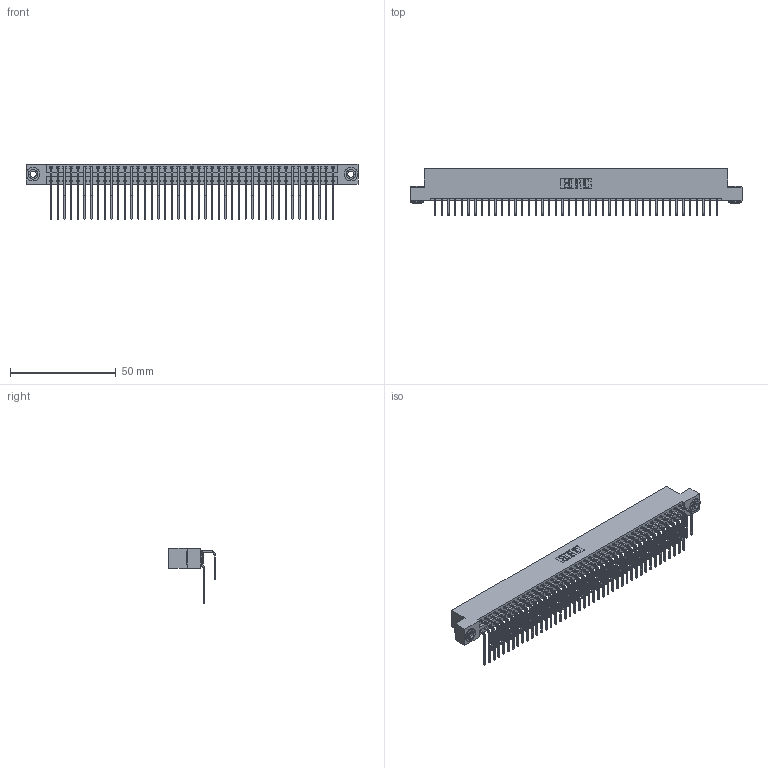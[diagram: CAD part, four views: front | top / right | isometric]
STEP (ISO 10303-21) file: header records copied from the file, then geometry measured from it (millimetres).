
FILE_DESCRIPTION (( 'STEP AP203' ), '1' );
FILE_NAME ('396-086-558-203.STEP', '2019-11-03T13:31:06', ( '' ), ( '' ), 'SwSTEP 2.0', 'SolidWorks 2016', '' );
FILE_SCHEMA (( 'CONFIG_CONTROL_DESIGN' ));
Length unit declared in the file: inch
Products named in the file (5): 345-292-001_558 Tail - 2; 345-250-002_345-250-002-102; 345-292-001_558 559 Tail - 1; 396-086-558-203; 346 Part_Flush Mounting Lugs - 0.156 Dia-TH
Assembly tree (89 placements, depth 2):
  396-086-558-203
    346 Part_Flush Mounting Lugs - 0.156 Dia-TH
    345-292-001_558 559 Tail - 1  x43
    345-292-001_558 Tail - 2  x43
    345-250-002_345-250-002-102  x2
Bounding box: 157.1 x 22.16 x 26.16 mm (x, y, z)
Volume: 15842.4 mm3; surface area: 24386.3 mm2
Topology: 89 solids, 89 shells, 4804 faces, 14251 edges, 9382 vertices
Faces by surface type: plane 3268, cylinder 1528, cone 8
Entity records: 30362 total; most frequent: CARTESIAN_POINT 5030, ORIENTED_EDGE 4906, DIRECTION 4487, EDGE_CURVE 2453, VECTOR 2085, LINE 2085, VERTEX_POINT 1630, AXIS2_PLACEMENT_3D 1201
